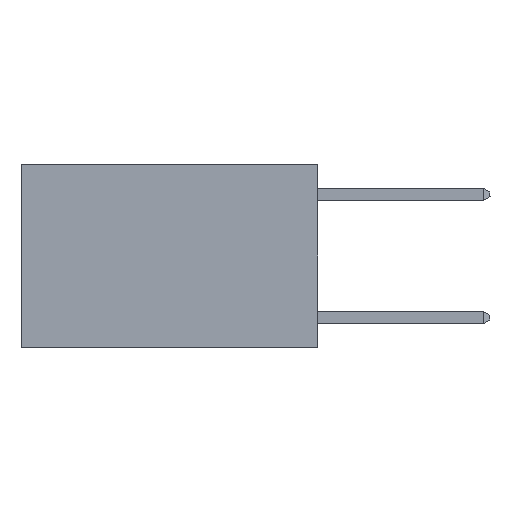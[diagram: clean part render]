
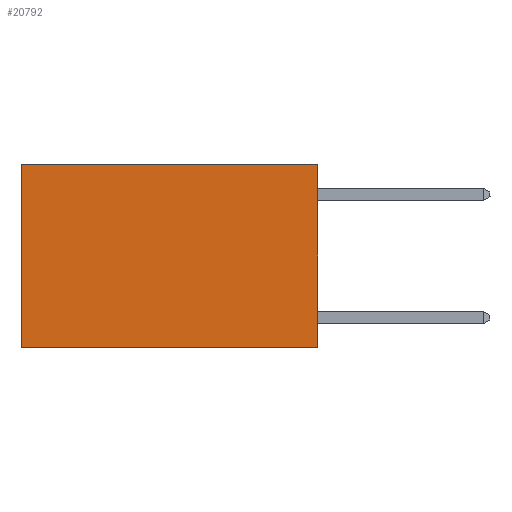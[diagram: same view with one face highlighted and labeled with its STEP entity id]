
A CAD part, left-side view. The second image highlights one B-rep face of the part: STEP entity #20792.
In plain terms, the highlighted planar face has unit normal (-1, 0, 0).
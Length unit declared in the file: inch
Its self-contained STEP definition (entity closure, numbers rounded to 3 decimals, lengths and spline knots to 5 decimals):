
#35 = EDGE_CURVE ( 'NONE', #8367, #13958, #19808, .T. ) ;
#74 = PLANE ( 'NONE',  #10662 ) ;
#538 = LINE ( 'NONE', #2752, #8224 ) ;
#1133 = EDGE_CURVE ( 'NONE', #16539, #13958, #4352, .T. ) ;
#1352 = VECTOR ( 'NONE', #14601, 39.37008 ) ;
#1659 = DIRECTION ( 'NONE',  ( 0., 1., 0. ) ) ;
#1675 = DIRECTION ( 'NONE',  ( 1., 0., 0. ) ) ;
#1702 = FACE_OUTER_BOUND ( 'NONE', #6143, .T. ) ;
#2323 = ORIENTED_EDGE ( 'NONE', *, *, #35, .T. ) ;
#2509 = LINE ( 'NONE', #22660, #1352 ) ;
#2752 = CARTESIAN_POINT ( 'NONE',  ( 0.2625, 0., 0. ) ) ;
#3233 = VECTOR ( 'NONE', #1659, 39.37008 ) ;
#4352 = LINE ( 'NONE', #4727, #3233 ) ;
#4727 = CARTESIAN_POINT ( 'NONE',  ( 0.2625, 0., -0.37 ) ) ;
#4928 = ORIENTED_EDGE ( 'NONE', *, *, #23239, .F. ) ;
#5959 = ORIENTED_EDGE ( 'NONE', *, *, #8479, .T. ) ;
#6143 = EDGE_LOOP ( 'NONE', ( #2323, #15273, #4928, #5959 ) ) ;
#6448 = DIRECTION ( 'NONE',  ( 0., 0., -1. ) ) ;
#8224 = VECTOR ( 'NONE', #6448, 39.37008 ) ;
#8367 = VERTEX_POINT ( 'NONE', #20073 ) ;
#8479 = EDGE_CURVE ( 'NONE', #18443, #8367, #2509, .T. ) ;
#8512 = CARTESIAN_POINT ( 'NONE',  ( 0.2625, 0., -0.37 ) ) ;
#10662 = AXIS2_PLACEMENT_3D ( 'NONE', #23468, #1675, #16197 ) ;
#13958 = VERTEX_POINT ( 'NONE', #19071 ) ;
#14601 = DIRECTION ( 'NONE',  ( 0., 1., 0. ) ) ;
#15228 = DIRECTION ( 'NONE',  ( 0., 0., -1. ) ) ;
#15243 = CARTESIAN_POINT ( 'NONE',  ( 0.2625, 0., 0. ) ) ;
#15273 = ORIENTED_EDGE ( 'NONE', *, *, #1133, .F. ) ;
#15792 = VECTOR ( 'NONE', #15228, 39.37008 ) ;
#16197 = DIRECTION ( 'NONE',  ( 0., 0., -1. ) ) ;
#16539 = VERTEX_POINT ( 'NONE', #8512 ) ;
#18443 = VERTEX_POINT ( 'NONE', #15243 ) ;
#19071 = CARTESIAN_POINT ( 'NONE',  ( 0.2625, 0.6, -0.37 ) ) ;
#19808 = LINE ( 'NONE', #20649, #15792 ) ;
#20073 = CARTESIAN_POINT ( 'NONE',  ( 0.2625, 0.6, 0. ) ) ;
#20649 = CARTESIAN_POINT ( 'NONE',  ( 0.2625, 0.6, 0. ) ) ;
#20792 = ADVANCED_FACE ( 'NONE', ( #1702 ), #74, .F. ) ;
#22660 = CARTESIAN_POINT ( 'NONE',  ( 0.2625, 0., 0. ) ) ;
#23239 = EDGE_CURVE ( 'NONE', #18443, #16539, #538, .T. ) ;
#23468 = CARTESIAN_POINT ( 'NONE',  ( 0.2625, 0., 0. ) ) ;
